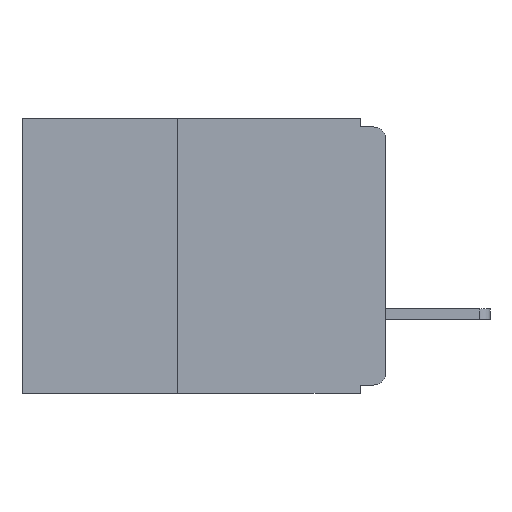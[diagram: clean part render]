
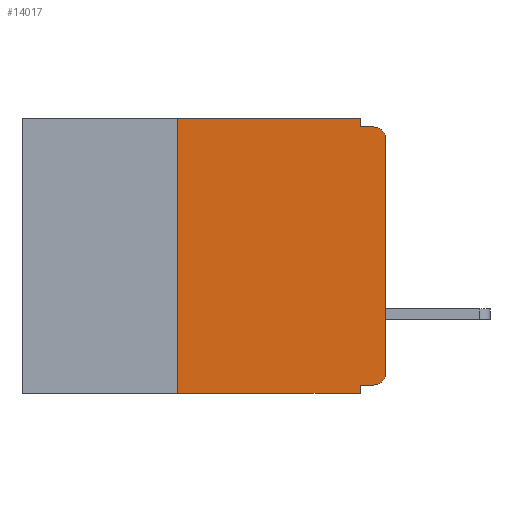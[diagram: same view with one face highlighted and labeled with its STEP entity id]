
A CAD part, left-side view. The second image highlights one B-rep face of the part: STEP entity #14017.
In plain terms, the highlighted planar face has unit normal (-1, 0, 0).
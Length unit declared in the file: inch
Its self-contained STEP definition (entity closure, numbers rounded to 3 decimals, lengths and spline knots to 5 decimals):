
#322 = EDGE_CURVE ( 'NONE', #1955, #16447, #11589, .T. ) ;
#346 = CARTESIAN_POINT ( 'NONE',  ( 0., 0.031, -0.01 ) ) ;
#1322 = EDGE_CURVE ( 'NONE', #7276, #18215, #9472, .T. ) ;
#1367 = CARTESIAN_POINT ( 'NONE',  ( 0., 0., 0. ) ) ;
#1544 = VERTEX_POINT ( 'NONE', #13704 ) ;
#1559 = DIRECTION ( 'NONE',  ( 0., -1., 0. ) ) ;
#1842 = VERTEX_POINT ( 'NONE', #2258 ) ;
#1955 = VERTEX_POINT ( 'NONE', #9594 ) ;
#2258 = CARTESIAN_POINT ( 'NONE',  ( 0., 0.015, -0.01 ) ) ;
#2842 = DIRECTION ( 'NONE',  ( -1., 0., 0. ) ) ;
#2959 = CARTESIAN_POINT ( 'NONE',  ( 0., 0.437, 0. ) ) ;
#2966 = AXIS2_PLACEMENT_3D ( 'NONE', #2959, #14871, #5903 ) ;
#3484 = DIRECTION ( 'NONE',  ( 0., 0., 1. ) ) ;
#3567 = EDGE_CURVE ( 'NONE', #1544, #12517, #3960, .T. ) ;
#3690 = DIRECTION ( 'NONE',  ( 0., -1., 0. ) ) ;
#3694 = VERTEX_POINT ( 'NONE', #12039 ) ;
#3720 = LINE ( 'NONE', #7430, #11213 ) ;
#3797 = CARTESIAN_POINT ( 'NONE',  ( 0., 0.015, -0.32 ) ) ;
#3960 = LINE ( 'NONE', #1367, #11932 ) ;
#4285 = EDGE_CURVE ( 'NONE', #12517, #1842, #6240, .T. ) ;
#4384 = AXIS2_PLACEMENT_3D ( 'NONE', #11782, #2842, #13260 ) ;
#5067 = CARTESIAN_POINT ( 'NONE',  ( 0., 0.437, -0.33 ) ) ;
#5322 = LINE ( 'NONE', #12642, #17281 ) ;
#5501 = VECTOR ( 'NONE', #16215, 39.37008 ) ;
#5903 = DIRECTION ( 'NONE',  ( 0., 0., -1. ) ) ;
#6015 = VERTEX_POINT ( 'NONE', #14929 ) ;
#6222 = CARTESIAN_POINT ( 'NONE',  ( 0., 0.031, 0. ) ) ;
#6240 = CIRCLE ( 'NONE', #16322, 0.015 ) ;
#6531 = ORIENTED_EDGE ( 'NONE', *, *, #13303, .F. ) ;
#6568 = DIRECTION ( 'NONE',  ( 0., -1., 0. ) ) ;
#6625 = VECTOR ( 'NONE', #3484, 39.37008 ) ;
#6946 = CARTESIAN_POINT ( 'NONE',  ( 0., 0.25, 0. ) ) ;
#7209 = DIRECTION ( 'NONE',  ( 0., 0., -1. ) ) ;
#7234 = DIRECTION ( 'NONE',  ( 0., 0., 1. ) ) ;
#7276 = VERTEX_POINT ( 'NONE', #6222 ) ;
#7430 = CARTESIAN_POINT ( 'NONE',  ( 0., 0., -0.01 ) ) ;
#7615 = DIRECTION ( 'NONE',  ( -1., 0., 0. ) ) ;
#8939 = EDGE_CURVE ( 'NONE', #18215, #1842, #3720, .T. ) ;
#9312 = VECTOR ( 'NONE', #7209, 39.37008 ) ;
#9472 = LINE ( 'NONE', #16371, #12497 ) ;
#9594 = CARTESIAN_POINT ( 'NONE',  ( 0., 0.25, -0.33 ) ) ;
#9601 = CARTESIAN_POINT ( 'NONE',  ( 0., 0., -0.025 ) ) ;
#9673 = ORIENTED_EDGE ( 'NONE', *, *, #13654, .T. ) ;
#10689 = ORIENTED_EDGE ( 'NONE', *, *, #4285, .T. ) ;
#10713 = EDGE_CURVE ( 'NONE', #13740, #1544, #14611, .T. ) ;
#10724 = ORIENTED_EDGE ( 'NONE', *, *, #322, .F. ) ;
#10930 = ORIENTED_EDGE ( 'NONE', *, *, #1322, .F. ) ;
#11213 = VECTOR ( 'NONE', #1559, 39.37008 ) ;
#11589 = LINE ( 'NONE', #17400, #6625 ) ;
#11782 = CARTESIAN_POINT ( 'NONE',  ( 0., 0.015, -0.305 ) ) ;
#11890 = PLANE ( 'NONE',  #2966 ) ;
#11932 = VECTOR ( 'NONE', #7234, 39.37008 ) ;
#12039 = CARTESIAN_POINT ( 'NONE',  ( 0., 0.031, -0.33 ) ) ;
#12497 = VECTOR ( 'NONE', #19281, 39.37008 ) ;
#12517 = VERTEX_POINT ( 'NONE', #9601 ) ;
#12642 = CARTESIAN_POINT ( 'NONE',  ( 0., 0.437, 0. ) ) ;
#12669 = EDGE_CURVE ( 'NONE', #6015, #3694, #17732, .T. ) ;
#13260 = DIRECTION ( 'NONE',  ( 0., 0., -1. ) ) ;
#13303 = EDGE_CURVE ( 'NONE', #13740, #6015, #13476, .T. ) ;
#13476 = LINE ( 'NONE', #14696, #5501 ) ;
#13654 = EDGE_CURVE ( 'NONE', #1955, #3694, #15340, .T. ) ;
#13704 = CARTESIAN_POINT ( 'NONE',  ( 0., 0., -0.305 ) ) ;
#13740 = VERTEX_POINT ( 'NONE', #3797 ) ;
#13743 = EDGE_LOOP ( 'NONE', ( #15277, #10689, #15412, #10930, #13887, #10724, #9673, #14515, #6531, #15003 ) ) ;
#13887 = ORIENTED_EDGE ( 'NONE', *, *, #18416, .F. ) ;
#14017 = ADVANCED_FACE ( 'NONE', ( #16250 ), #11890, .F. ) ;
#14515 = ORIENTED_EDGE ( 'NONE', *, *, #12669, .F. ) ;
#14611 = CIRCLE ( 'NONE', #4384, 0.015 ) ;
#14659 = CARTESIAN_POINT ( 'NONE',  ( 0., 0.031, -0.33 ) ) ;
#14696 = CARTESIAN_POINT ( 'NONE',  ( 0., 0., -0.32 ) ) ;
#14853 = VECTOR ( 'NONE', #6568, 39.37008 ) ;
#14871 = DIRECTION ( 'NONE',  ( 1., 0., 0. ) ) ;
#14929 = CARTESIAN_POINT ( 'NONE',  ( 0., 0.031, -0.32 ) ) ;
#15003 = ORIENTED_EDGE ( 'NONE', *, *, #10713, .T. ) ;
#15277 = ORIENTED_EDGE ( 'NONE', *, *, #3567, .T. ) ;
#15340 = LINE ( 'NONE', #5067, #14853 ) ;
#15412 = ORIENTED_EDGE ( 'NONE', *, *, #8939, .F. ) ;
#16215 = DIRECTION ( 'NONE',  ( 0., 1., 0. ) ) ;
#16250 = FACE_OUTER_BOUND ( 'NONE', #13743, .T. ) ;
#16322 = AXIS2_PLACEMENT_3D ( 'NONE', #16557, #7615, #18094 ) ;
#16371 = CARTESIAN_POINT ( 'NONE',  ( 0., 0.031, 0. ) ) ;
#16447 = VERTEX_POINT ( 'NONE', #6946 ) ;
#16557 = CARTESIAN_POINT ( 'NONE',  ( 0., 0.015, -0.025 ) ) ;
#17281 = VECTOR ( 'NONE', #3690, 39.37008 ) ;
#17400 = CARTESIAN_POINT ( 'NONE',  ( 0., 0.25, -0.33 ) ) ;
#17732 = LINE ( 'NONE', #14659, #9312 ) ;
#18094 = DIRECTION ( 'NONE',  ( 0., 0., -1. ) ) ;
#18215 = VERTEX_POINT ( 'NONE', #346 ) ;
#18416 = EDGE_CURVE ( 'NONE', #16447, #7276, #5322, .T. ) ;
#19281 = DIRECTION ( 'NONE',  ( 0., 0., -1. ) ) ;
